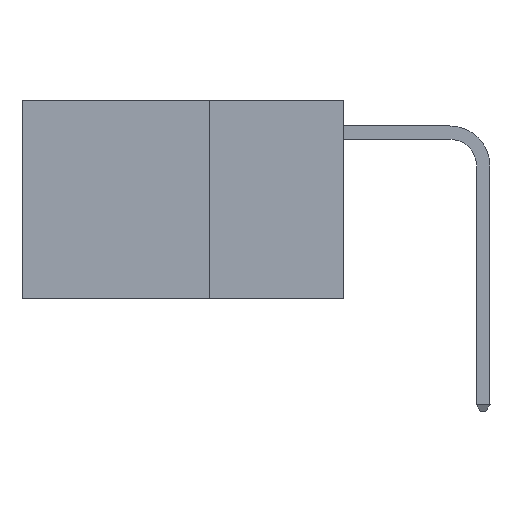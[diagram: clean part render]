
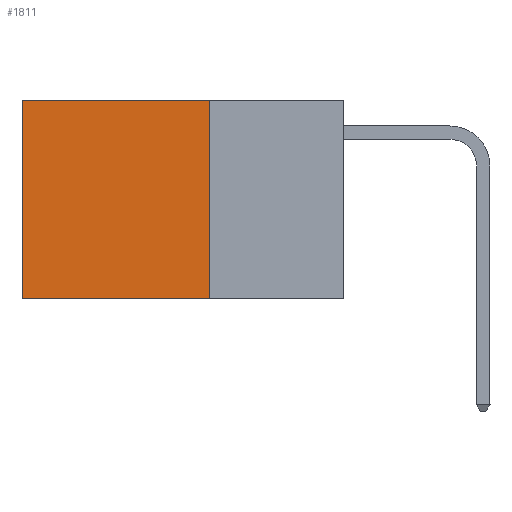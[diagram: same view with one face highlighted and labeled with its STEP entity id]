
A CAD part, left-side view. The second image highlights one B-rep face of the part: STEP entity #1811.
In plain terms, the highlighted planar face has unit normal (-1, 0, 0).
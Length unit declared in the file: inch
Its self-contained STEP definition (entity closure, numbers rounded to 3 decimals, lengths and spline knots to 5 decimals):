
#10 = CARTESIAN_POINT ( 'NONE',  ( 0.2625, 0.25, 0. ) ) ;
#209 = PLANE ( 'NONE',  #6021 ) ;
#463 = VERTEX_POINT ( 'NONE', #15591 ) ;
#903 = CARTESIAN_POINT ( 'NONE',  ( 0.2625, 0.6, -0.37 ) ) ;
#1233 = EDGE_CURVE ( 'NONE', #10246, #3883, #15277, .T. ) ;
#1681 = VECTOR ( 'NONE', #9905, 39.37008 ) ;
#1811 = ADVANCED_FACE ( 'NONE', ( #2038 ), #209, .F. ) ;
#1851 = EDGE_CURVE ( 'NONE', #463, #5287, #15447, .T. ) ;
#2038 = FACE_OUTER_BOUND ( 'NONE', #9750, .T. ) ;
#2808 = EDGE_CURVE ( 'NONE', #5287, #3883, #3392, .T. ) ;
#3392 = LINE ( 'NONE', #6071, #1681 ) ;
#3883 = VERTEX_POINT ( 'NONE', #903 ) ;
#4856 = VECTOR ( 'NONE', #14970, 39.37008 ) ;
#5040 = VECTOR ( 'NONE', #13714, 39.37008 ) ;
#5287 = VERTEX_POINT ( 'NONE', #6171 ) ;
#6021 = AXIS2_PLACEMENT_3D ( 'NONE', #10, #13723, #13281 ) ;
#6071 = CARTESIAN_POINT ( 'NONE',  ( 0.2625, 0.6, 0. ) ) ;
#6171 = CARTESIAN_POINT ( 'NONE',  ( 0.2625, 0.6, 0. ) ) ;
#6697 = ORIENTED_EDGE ( 'NONE', *, *, #1851, .T. ) ;
#7546 = VECTOR ( 'NONE', #7795, 39.37008 ) ;
#7795 = DIRECTION ( 'NONE',  ( 0., 0., -1. ) ) ;
#7927 = LINE ( 'NONE', #14052, #7546 ) ;
#8245 = ORIENTED_EDGE ( 'NONE', *, *, #2808, .T. ) ;
#9552 = ORIENTED_EDGE ( 'NONE', *, *, #15870, .F. ) ;
#9750 = EDGE_LOOP ( 'NONE', ( #8245, #11386, #9552, #6697 ) ) ;
#9905 = DIRECTION ( 'NONE',  ( 0., 0., -1. ) ) ;
#10246 = VERTEX_POINT ( 'NONE', #14622 ) ;
#11386 = ORIENTED_EDGE ( 'NONE', *, *, #1233, .F. ) ;
#13281 = DIRECTION ( 'NONE',  ( 0., 0., -1. ) ) ;
#13714 = DIRECTION ( 'NONE',  ( 0., 1., 0. ) ) ;
#13723 = DIRECTION ( 'NONE',  ( 1., 0., 0. ) ) ;
#13813 = CARTESIAN_POINT ( 'NONE',  ( 0.2625, 0.25, 0. ) ) ;
#14052 = CARTESIAN_POINT ( 'NONE',  ( 0.2625, 0.25, 0. ) ) ;
#14622 = CARTESIAN_POINT ( 'NONE',  ( 0.2625, 0.25, -0.37 ) ) ;
#14970 = DIRECTION ( 'NONE',  ( 0., 1., 0. ) ) ;
#15018 = CARTESIAN_POINT ( 'NONE',  ( 0.2625, 0.25, -0.37 ) ) ;
#15277 = LINE ( 'NONE', #15018, #4856 ) ;
#15447 = LINE ( 'NONE', #13813, #5040 ) ;
#15591 = CARTESIAN_POINT ( 'NONE',  ( 0.2625, 0.25, 0. ) ) ;
#15870 = EDGE_CURVE ( 'NONE', #463, #10246, #7927, .T. ) ;
